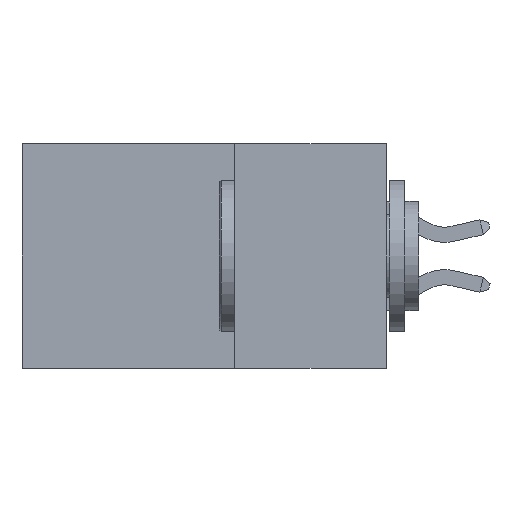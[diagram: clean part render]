
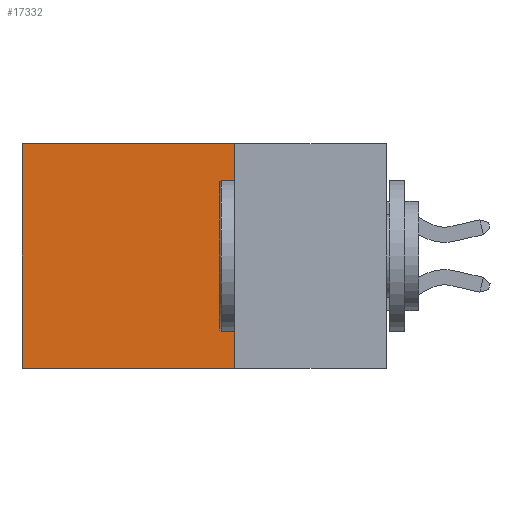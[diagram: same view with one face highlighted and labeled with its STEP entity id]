
A CAD part, left-side view. The second image highlights one B-rep face of the part: STEP entity #17332.
In plain terms, the highlighted planar face has unit normal (-1, 0, 0).
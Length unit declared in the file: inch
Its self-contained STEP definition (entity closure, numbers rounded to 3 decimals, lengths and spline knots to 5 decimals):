
#49 = DIRECTION ( 'NONE',  ( 0., 1., 0. ) ) ;
#365 = FACE_OUTER_BOUND ( 'NONE', #22043, .T. ) ;
#1586 = CARTESIAN_POINT ( 'NONE',  ( 0.298, 0.25, 0. ) ) ;
#2298 = CARTESIAN_POINT ( 'NONE',  ( 0.298, 0.6, 0. ) ) ;
#2989 = CARTESIAN_POINT ( 'NONE',  ( 0.298, 0.6, -0.37 ) ) ;
#3415 = EDGE_CURVE ( 'NONE', #22392, #21184, #8855, .T. ) ;
#4919 = DIRECTION ( 'NONE',  ( 0., 0., -1. ) ) ;
#5166 = DIRECTION ( 'NONE',  ( 1., 0., 0. ) ) ;
#5217 = LINE ( 'NONE', #9721, #15801 ) ;
#5864 = ORIENTED_EDGE ( 'NONE', *, *, #3415, .F. ) ;
#6569 = ORIENTED_EDGE ( 'NONE', *, *, #14813, .T. ) ;
#6959 = VECTOR ( 'NONE', #20722, 39.37008 ) ;
#8628 = CARTESIAN_POINT ( 'NONE',  ( 0.298, 0.25, -0.37 ) ) ;
#8855 = LINE ( 'NONE', #8628, #6959 ) ;
#9150 = VECTOR ( 'NONE', #11375, 39.37008 ) ;
#9721 = CARTESIAN_POINT ( 'NONE',  ( 0.298, 0.6, 0. ) ) ;
#10917 = AXIS2_PLACEMENT_3D ( 'NONE', #1586, #5166, #4919 ) ;
#11375 = DIRECTION ( 'NONE',  ( 0., 0., -1. ) ) ;
#11459 = EDGE_CURVE ( 'NONE', #16825, #22392, #12943, .T. ) ;
#11616 = ORIENTED_EDGE ( 'NONE', *, *, #20895, .T. ) ;
#11916 = CARTESIAN_POINT ( 'NONE',  ( 0.298, 0.25, 0. ) ) ;
#12943 = LINE ( 'NONE', #13119, #9150 ) ;
#13119 = CARTESIAN_POINT ( 'NONE',  ( 0.298, 0.25, 0. ) ) ;
#14566 = ORIENTED_EDGE ( 'NONE', *, *, #11459, .F. ) ;
#14813 = EDGE_CURVE ( 'NONE', #15993, #21184, #5217, .T. ) ;
#15404 = PLANE ( 'NONE',  #10917 ) ;
#15801 = VECTOR ( 'NONE', #21619, 39.37008 ) ;
#15993 = VERTEX_POINT ( 'NONE', #2298 ) ;
#16825 = VERTEX_POINT ( 'NONE', #18849 ) ;
#17332 = ADVANCED_FACE ( 'NONE', ( #365 ), #15404, .F. ) ;
#18849 = CARTESIAN_POINT ( 'NONE',  ( 0.298, 0.25, 0. ) ) ;
#19197 = LINE ( 'NONE', #11916, #19715 ) ;
#19715 = VECTOR ( 'NONE', #49, 39.37008 ) ;
#20437 = CARTESIAN_POINT ( 'NONE',  ( 0.298, 0.25, -0.37 ) ) ;
#20722 = DIRECTION ( 'NONE',  ( 0., 1., 0. ) ) ;
#20895 = EDGE_CURVE ( 'NONE', #16825, #15993, #19197, .T. ) ;
#21184 = VERTEX_POINT ( 'NONE', #2989 ) ;
#21619 = DIRECTION ( 'NONE',  ( 0., 0., -1. ) ) ;
#22043 = EDGE_LOOP ( 'NONE', ( #6569, #5864, #14566, #11616 ) ) ;
#22392 = VERTEX_POINT ( 'NONE', #20437 ) ;
